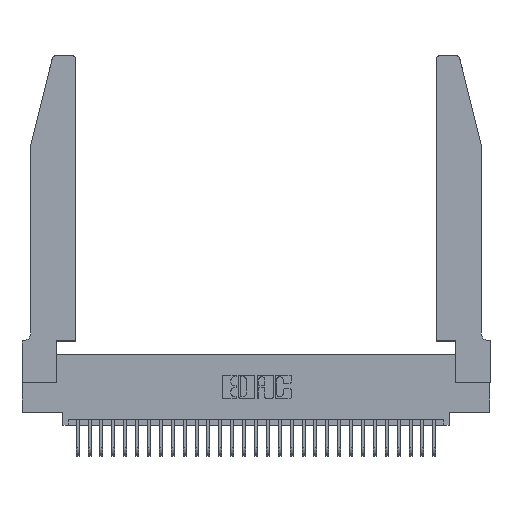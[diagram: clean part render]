
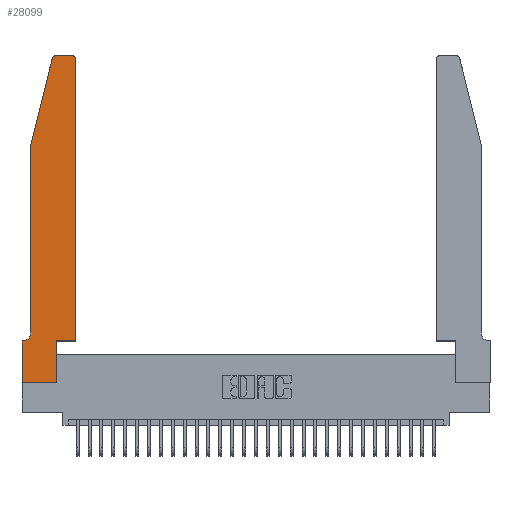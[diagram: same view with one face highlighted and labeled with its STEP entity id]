
A CAD part, top view. The second image highlights one B-rep face of the part: STEP entity #28099.
In plain terms, the highlighted planar face has unit normal (0, 0, 1).
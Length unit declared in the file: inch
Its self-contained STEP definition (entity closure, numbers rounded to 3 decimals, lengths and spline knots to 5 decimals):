
#28 = CARTESIAN_POINT ( 'NONE',  ( 0.0755, 0.35, 0.37 ) ) ;
#438 = VERTEX_POINT ( 'NONE', #8471 ) ;
#458 = CARTESIAN_POINT ( 'NONE',  ( 0.4505, 0.35, 0.37 ) ) ;
#599 = EDGE_CURVE ( 'NONE', #438, #30254, #8860, .T. ) ;
#894 = CARTESIAN_POINT ( 'NONE',  ( 0.2865, 0., 0.37 ) ) ;
#952 = DIRECTION ( 'NONE',  ( 0., -1., 0. ) ) ;
#1231 = EDGE_CURVE ( 'NONE', #26832, #17179, #16662, .T. ) ;
#1299 = EDGE_CURVE ( 'NONE', #5036, #18165, #28357, .T. ) ;
#1430 = ORIENTED_EDGE ( 'NONE', *, *, #599, .T. ) ;
#1549 = VECTOR ( 'NONE', #15179, 39.37008 ) ;
#1712 = VECTOR ( 'NONE', #23226, 39.37008 ) ;
#1863 = DIRECTION ( 'NONE',  ( 0., -1., 0. ) ) ;
#2319 = DIRECTION ( 'NONE',  ( 1., 0., 0. ) ) ;
#2322 = CARTESIAN_POINT ( 'NONE',  ( 0.0055, 0.35, 0.37 ) ) ;
#2881 = CARTESIAN_POINT ( 'NONE',  ( 0., 0., 0.37 ) ) ;
#3355 = CARTESIAN_POINT ( 'NONE',  ( 0., 0.35, 0.37 ) ) ;
#3545 = AXIS2_PLACEMENT_3D ( 'NONE', #3355, #8399, #25875 ) ;
#4051 = CARTESIAN_POINT ( 'NONE',  ( 0.0055, 0.42, 0.37 ) ) ;
#4098 = VECTOR ( 'NONE', #17737, 39.37008 ) ;
#4146 = VERTEX_POINT ( 'NONE', #29011 ) ;
#4177 = VECTOR ( 'NONE', #8161, 39.37008 ) ;
#4410 = EDGE_CURVE ( 'NONE', #30130, #4146, #12861, .T. ) ;
#4769 = DIRECTION ( 'NONE',  ( -1., 0., 0. ) ) ;
#4986 = CARTESIAN_POINT ( 'NONE',  ( 0.0755, 2., 0.37 ) ) ;
#5036 = VERTEX_POINT ( 'NONE', #12279 ) ;
#5406 = AXIS2_PLACEMENT_3D ( 'NONE', #7656, #25148, #10193 ) ;
#5747 = VERTEX_POINT ( 'NONE', #30801 ) ;
#5884 = PLANE ( 'NONE',  #3545 ) ;
#6748 = EDGE_CURVE ( 'NONE', #30254, #26832, #24376, .T. ) ;
#6798 = CARTESIAN_POINT ( 'NONE',  ( 0.4205, 2.72, 0.37 ) ) ;
#6896 = CARTESIAN_POINT ( 'NONE',  ( 0.2865, 0.35, 0.37 ) ) ;
#7204 = FACE_OUTER_BOUND ( 'NONE', #30063, .T. ) ;
#7318 = ORIENTED_EDGE ( 'NONE', *, *, #11828, .T. ) ;
#7656 = CARTESIAN_POINT ( 'NONE',  ( 0.284, 2.72, 0.37 ) ) ;
#8161 = DIRECTION ( 'NONE',  ( -1., 0., 0. ) ) ;
#8235 = CARTESIAN_POINT ( 'NONE',  ( 0.4505, 0.35, 0.37 ) ) ;
#8242 = LINE ( 'NONE', #28, #1549 ) ;
#8399 = DIRECTION ( 'NONE',  ( 0., 0., 1. ) ) ;
#8471 = CARTESIAN_POINT ( 'NONE',  ( 0., 0.35, 0.37 ) ) ;
#8472 = EDGE_CURVE ( 'NONE', #18165, #438, #8242, .T. ) ;
#8860 = LINE ( 'NONE', #2881, #14737 ) ;
#9179 = VERTEX_POINT ( 'NONE', #15699 ) ;
#9267 = ORIENTED_EDGE ( 'NONE', *, *, #1299, .T. ) ;
#9333 = DIRECTION ( 'NONE',  ( 1., 0., 0. ) ) ;
#9339 = CARTESIAN_POINT ( 'NONE',  ( 0.0755, 2., 0.37 ) ) ;
#9703 = CARTESIAN_POINT ( 'NONE',  ( 0.284, 2.75, 0.37 ) ) ;
#9714 = EDGE_CURVE ( 'NONE', #28270, #30130, #31944, .T. ) ;
#10106 = ORIENTED_EDGE ( 'NONE', *, *, #6748, .T. ) ;
#10193 = DIRECTION ( 'NONE',  ( 1., 0., 0. ) ) ;
#10452 = ORIENTED_EDGE ( 'NONE', *, *, #4410, .T. ) ;
#10517 = EDGE_CURVE ( 'NONE', #5747, #28270, #10872, .T. ) ;
#10757 = EDGE_CURVE ( 'NONE', #4146, #5036, #12939, .T. ) ;
#10872 = LINE ( 'NONE', #13112, #4177 ) ;
#11828 = EDGE_CURVE ( 'NONE', #25143, #9179, #19862, .T. ) ;
#12279 = CARTESIAN_POINT ( 'NONE',  ( 0.0755, 0.42, 0.37 ) ) ;
#12587 = CARTESIAN_POINT ( 'NONE',  ( 0.4505, 0.35, 0.37 ) ) ;
#12861 = LINE ( 'NONE', #4986, #13630 ) ;
#12939 = LINE ( 'NONE', #9339, #31234 ) ;
#13112 = CARTESIAN_POINT ( 'NONE',  ( 0.2605, 2.75, 0.37 ) ) ;
#13630 = VECTOR ( 'NONE', #19950, 39.37008 ) ;
#14737 = VECTOR ( 'NONE', #952, 39.37008 ) ;
#14835 = CARTESIAN_POINT ( 'NONE',  ( 0., 0., 0.37 ) ) ;
#15080 = LINE ( 'NONE', #8235, #1712 ) ;
#15179 = DIRECTION ( 'NONE',  ( -1., 0., 0. ) ) ;
#15551 = ORIENTED_EDGE ( 'NONE', *, *, #9714, .T. ) ;
#15699 = CARTESIAN_POINT ( 'NONE',  ( 0.4505, 2.72, 0.37 ) ) ;
#16662 = LINE ( 'NONE', #6896, #4098 ) ;
#16769 = ORIENTED_EDGE ( 'NONE', *, *, #1231, .T. ) ;
#17179 = VERTEX_POINT ( 'NONE', #18612 ) ;
#17653 = AXIS2_PLACEMENT_3D ( 'NONE', #4051, #29073, #4769 ) ;
#17737 = DIRECTION ( 'NONE',  ( 0., 1., 0. ) ) ;
#18165 = VERTEX_POINT ( 'NONE', #2322 ) ;
#18612 = CARTESIAN_POINT ( 'NONE',  ( 0.2865, 0.35, 0.37 ) ) ;
#18674 = ORIENTED_EDGE ( 'NONE', *, *, #10757, .T. ) ;
#19447 = AXIS2_PLACEMENT_3D ( 'NONE', #6798, #24293, #9333 ) ;
#19862 = LINE ( 'NONE', #12587, #32312 ) ;
#19950 = DIRECTION ( 'NONE',  ( -0.239, -0.971, 0. ) ) ;
#20093 = DIRECTION ( 'NONE',  ( 0., 1., 0. ) ) ;
#20638 = ORIENTED_EDGE ( 'NONE', *, *, #27056, .T. ) ;
#23226 = DIRECTION ( 'NONE',  ( 1., 0., 0. ) ) ;
#24293 = DIRECTION ( 'NONE',  ( 0., 0., 1. ) ) ;
#24376 = LINE ( 'NONE', #14835, #30216 ) ;
#24928 = ORIENTED_EDGE ( 'NONE', *, *, #8472, .T. ) ;
#25143 = VERTEX_POINT ( 'NONE', #458 ) ;
#25148 = DIRECTION ( 'NONE',  ( 0., 0., 1. ) ) ;
#25679 = ORIENTED_EDGE ( 'NONE', *, *, #10517, .T. ) ;
#25875 = DIRECTION ( 'NONE',  ( 1., 0., 0. ) ) ;
#26051 = CIRCLE ( 'NONE', #19447, 0.03 ) ;
#26832 = VERTEX_POINT ( 'NONE', #894 ) ;
#27056 = EDGE_CURVE ( 'NONE', #9179, #5747, #26051, .T. ) ;
#27492 = CARTESIAN_POINT ( 'NONE',  ( 0.25487, 2.72718, 0.37 ) ) ;
#28099 = ADVANCED_FACE ( 'NONE', ( #7204 ), #5884, .T. ) ;
#28270 = VERTEX_POINT ( 'NONE', #9703 ) ;
#28357 = CIRCLE ( 'NONE', #17653, 0.07 ) ;
#29011 = CARTESIAN_POINT ( 'NONE',  ( 0.0755, 2., 0.37 ) ) ;
#29073 = DIRECTION ( 'NONE',  ( 0., 0., -1. ) ) ;
#30063 = EDGE_LOOP ( 'NONE', ( #25679, #15551, #10452, #18674, #9267, #24928, #1430, #10106, #16769, #30752, #7318, #20638 ) ) ;
#30130 = VERTEX_POINT ( 'NONE', #27492 ) ;
#30216 = VECTOR ( 'NONE', #2319, 39.37008 ) ;
#30254 = VERTEX_POINT ( 'NONE', #30529 ) ;
#30529 = CARTESIAN_POINT ( 'NONE',  ( 0., 0., 0.37 ) ) ;
#30752 = ORIENTED_EDGE ( 'NONE', *, *, #30963, .T. ) ;
#30801 = CARTESIAN_POINT ( 'NONE',  ( 0.4205, 2.75, 0.37 ) ) ;
#30963 = EDGE_CURVE ( 'NONE', #17179, #25143, #15080, .T. ) ;
#31234 = VECTOR ( 'NONE', #1863, 39.37008 ) ;
#31944 = CIRCLE ( 'NONE', #5406, 0.03 ) ;
#32312 = VECTOR ( 'NONE', #20093, 39.37008 ) ;
